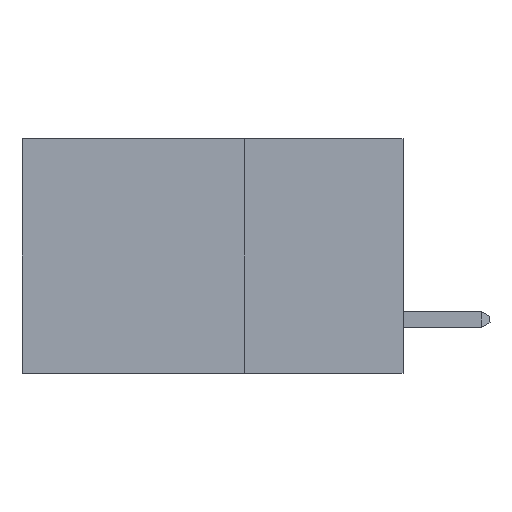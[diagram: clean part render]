
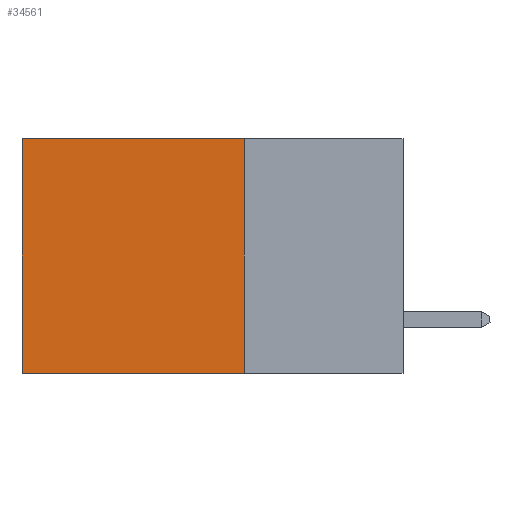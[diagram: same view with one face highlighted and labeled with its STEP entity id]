
A CAD part, left-side view. The second image highlights one B-rep face of the part: STEP entity #34561.
In plain terms, the highlighted planar face has unit normal (-1, 0, 0).
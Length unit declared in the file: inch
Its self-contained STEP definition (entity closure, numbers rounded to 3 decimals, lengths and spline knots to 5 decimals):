
#766 = VECTOR ( 'NONE', #36933, 39.37008 ) ;
#2009 = CARTESIAN_POINT ( 'NONE',  ( 0.2875, 0.6, 0. ) ) ;
#3593 = AXIS2_PLACEMENT_3D ( 'NONE', #14192, #34596, #17303 ) ;
#4529 = DIRECTION ( 'NONE',  ( 0., 1., 0. ) ) ;
#8292 = VECTOR ( 'NONE', #35453, 39.37008 ) ;
#9965 = CARTESIAN_POINT ( 'NONE',  ( 0.2875, 0.6, 0. ) ) ;
#10983 = EDGE_CURVE ( 'NONE', #15806, #35501, #20720, .T. ) ;
#11241 = ORIENTED_EDGE ( 'NONE', *, *, #28396, .F. ) ;
#11934 = EDGE_LOOP ( 'NONE', ( #30691, #11241, #35293, #12713 ) ) ;
#12713 = ORIENTED_EDGE ( 'NONE', *, *, #19611, .T. ) ;
#12749 = CARTESIAN_POINT ( 'NONE',  ( 0.2875, 0.25, 0. ) ) ;
#13479 = VERTEX_POINT ( 'NONE', #31115 ) ;
#14192 = CARTESIAN_POINT ( 'NONE',  ( 0.2875, 0.25, 0. ) ) ;
#15269 = VERTEX_POINT ( 'NONE', #9965 ) ;
#15806 = VERTEX_POINT ( 'NONE', #12749 ) ;
#17303 = DIRECTION ( 'NONE',  ( 0., 0., -1. ) ) ;
#18096 = FACE_OUTER_BOUND ( 'NONE', #11934, .T. ) ;
#19336 = DIRECTION ( 'NONE',  ( 0., 0., -1. ) ) ;
#19611 = EDGE_CURVE ( 'NONE', #15806, #15269, #35198, .T. ) ;
#20720 = LINE ( 'NONE', #33712, #36043 ) ;
#23893 = CARTESIAN_POINT ( 'NONE',  ( 0.2875, 0.25, -0.37 ) ) ;
#27541 = VECTOR ( 'NONE', #4529, 39.37008 ) ;
#27800 = CARTESIAN_POINT ( 'NONE',  ( 0.2875, 0.25, 0. ) ) ;
#28396 = EDGE_CURVE ( 'NONE', #35501, #13479, #31503, .T. ) ;
#30691 = ORIENTED_EDGE ( 'NONE', *, *, #30746, .T. ) ;
#30746 = EDGE_CURVE ( 'NONE', #15269, #13479, #31793, .T. ) ;
#31115 = CARTESIAN_POINT ( 'NONE',  ( 0.2875, 0.6, -0.37 ) ) ;
#31503 = LINE ( 'NONE', #23893, #8292 ) ;
#31699 = PLANE ( 'NONE',  #3593 ) ;
#31793 = LINE ( 'NONE', #2009, #766 ) ;
#32212 = CARTESIAN_POINT ( 'NONE',  ( 0.2875, 0.25, -0.37 ) ) ;
#33712 = CARTESIAN_POINT ( 'NONE',  ( 0.2875, 0.25, 0. ) ) ;
#34561 = ADVANCED_FACE ( 'NONE', ( #18096 ), #31699, .F. ) ;
#34596 = DIRECTION ( 'NONE',  ( 1., 0., 0. ) ) ;
#35198 = LINE ( 'NONE', #27800, #27541 ) ;
#35293 = ORIENTED_EDGE ( 'NONE', *, *, #10983, .F. ) ;
#35453 = DIRECTION ( 'NONE',  ( 0., 1., 0. ) ) ;
#35501 = VERTEX_POINT ( 'NONE', #32212 ) ;
#36043 = VECTOR ( 'NONE', #19336, 39.37008 ) ;
#36933 = DIRECTION ( 'NONE',  ( 0., 0., -1. ) ) ;
